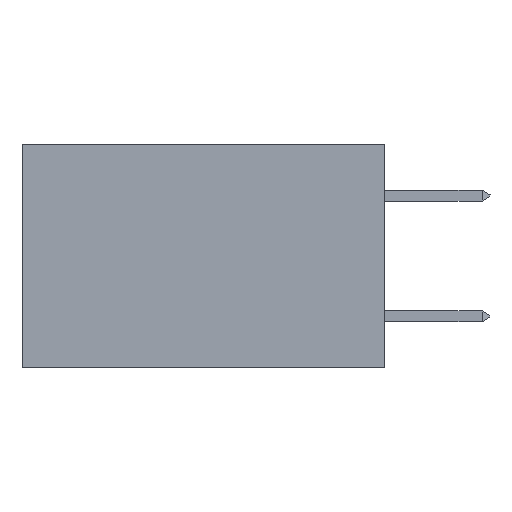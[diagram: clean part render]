
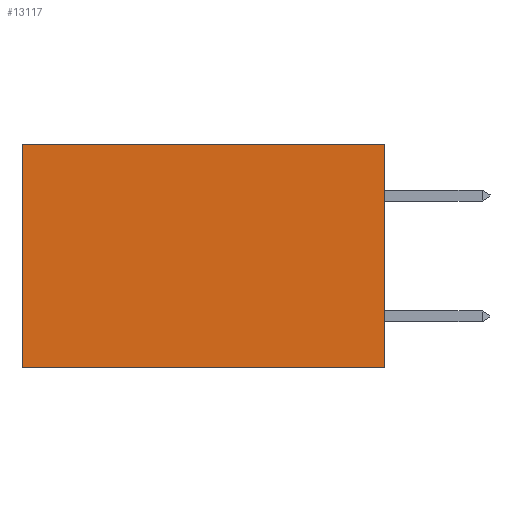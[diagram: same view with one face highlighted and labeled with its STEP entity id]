
A CAD part, left-side view. The second image highlights one B-rep face of the part: STEP entity #13117.
In plain terms, the highlighted planar face has unit normal (-1, 0, 0).
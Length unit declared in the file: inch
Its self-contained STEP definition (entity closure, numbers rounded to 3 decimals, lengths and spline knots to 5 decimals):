
#1413 = DIRECTION ( 'NONE',  ( 0., 0., -1. ) ) ;
#1582 = VERTEX_POINT ( 'NONE', #19846 ) ;
#2645 = ORIENTED_EDGE ( 'NONE', *, *, #5095, .F. ) ;
#3015 = CARTESIAN_POINT ( 'NONE',  ( 0.2875, 0., -0.37 ) ) ;
#3274 = DIRECTION ( 'NONE',  ( 1., 0., 0. ) ) ;
#3759 = VERTEX_POINT ( 'NONE', #8360 ) ;
#4151 = VECTOR ( 'NONE', #8213, 39.37008 ) ;
#4545 = VECTOR ( 'NONE', #6523, 39.37008 ) ;
#5095 = EDGE_CURVE ( 'NONE', #1582, #12935, #19372, .T. ) ;
#6104 = VECTOR ( 'NONE', #11503, 39.37008 ) ;
#6281 = CARTESIAN_POINT ( 'NONE',  ( 0.2875, 0., 0. ) ) ;
#6523 = DIRECTION ( 'NONE',  ( 0., 0., -1. ) ) ;
#7798 = DIRECTION ( 'NONE',  ( 0., 1., 0. ) ) ;
#8054 = EDGE_CURVE ( 'NONE', #13471, #1582, #19467, .T. ) ;
#8213 = DIRECTION ( 'NONE',  ( 0., 1., 0. ) ) ;
#8345 = AXIS2_PLACEMENT_3D ( 'NONE', #17922, #3274, #1413 ) ;
#8360 = CARTESIAN_POINT ( 'NONE',  ( 0.2875, 0.6, 0. ) ) ;
#8587 = LINE ( 'NONE', #6281, #12626 ) ;
#11250 = EDGE_LOOP ( 'NONE', ( #13974, #2645, #18027, #23502 ) ) ;
#11503 = DIRECTION ( 'NONE',  ( 0., 0., -1. ) ) ;
#12626 = VECTOR ( 'NONE', #7798, 39.37008 ) ;
#12935 = VERTEX_POINT ( 'NONE', #13423 ) ;
#13117 = ADVANCED_FACE ( 'NONE', ( #14346 ), #19781, .F. ) ;
#13423 = CARTESIAN_POINT ( 'NONE',  ( 0.2875, 0.6, -0.37 ) ) ;
#13471 = VERTEX_POINT ( 'NONE', #20656 ) ;
#13898 = CARTESIAN_POINT ( 'NONE',  ( 0.2875, 0., 0. ) ) ;
#13974 = ORIENTED_EDGE ( 'NONE', *, *, #22451, .T. ) ;
#14346 = FACE_OUTER_BOUND ( 'NONE', #11250, .T. ) ;
#15136 = CARTESIAN_POINT ( 'NONE',  ( 0.2875, 0.6, 0. ) ) ;
#16450 = LINE ( 'NONE', #15136, #6104 ) ;
#17922 = CARTESIAN_POINT ( 'NONE',  ( 0.2875, 0., 0. ) ) ;
#18027 = ORIENTED_EDGE ( 'NONE', *, *, #8054, .F. ) ;
#19213 = EDGE_CURVE ( 'NONE', #13471, #3759, #8587, .T. ) ;
#19372 = LINE ( 'NONE', #3015, #4151 ) ;
#19467 = LINE ( 'NONE', #13898, #4545 ) ;
#19781 = PLANE ( 'NONE',  #8345 ) ;
#19846 = CARTESIAN_POINT ( 'NONE',  ( 0.2875, 0., -0.37 ) ) ;
#20656 = CARTESIAN_POINT ( 'NONE',  ( 0.2875, 0., 0. ) ) ;
#22451 = EDGE_CURVE ( 'NONE', #3759, #12935, #16450, .T. ) ;
#23502 = ORIENTED_EDGE ( 'NONE', *, *, #19213, .T. ) ;
